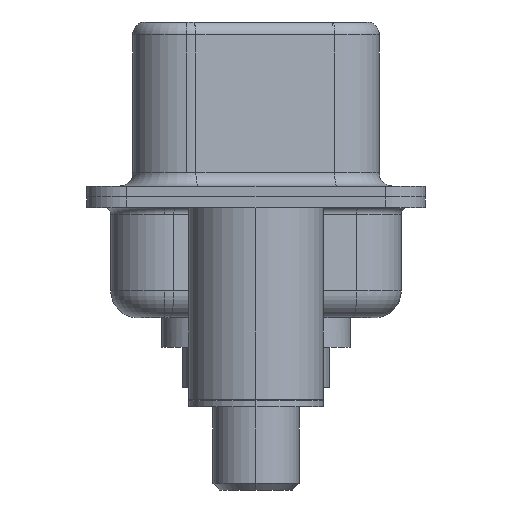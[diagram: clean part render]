
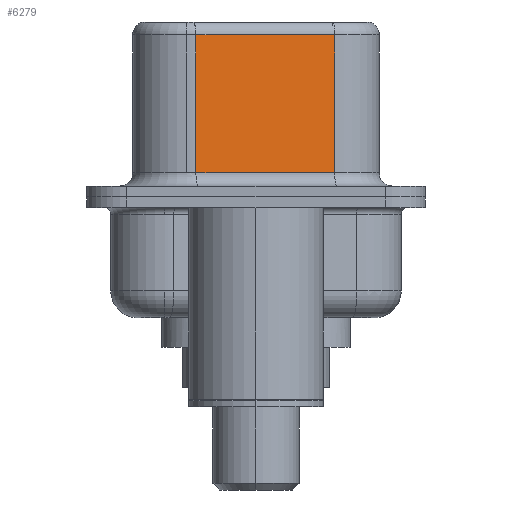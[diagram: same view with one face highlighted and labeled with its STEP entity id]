
A CAD part, left-side view. The second image highlights one B-rep face of the part: STEP entity #6279.
In plain terms, the highlighted planar face has unit normal (-0.985, -0.174, 0).
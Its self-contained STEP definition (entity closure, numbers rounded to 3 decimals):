
#723 = ORIENTED_EDGE ( 'NONE', *, *, #12810, .T. ) ;
#976 = AXIS2_PLACEMENT_3D ( 'NONE', #3949, #3891, #9021 ) ;
#1210 = CARTESIAN_POINT ( 'NONE',  ( 3.67, 2.233, 6.52 ) ) ;
#2506 = EDGE_LOOP ( 'NONE', ( #10487, #8328, #10010, #723 ) ) ;
#3475 = VECTOR ( 'NONE', #10980, 1000. ) ;
#3891 = DIRECTION ( 'NONE',  ( 0.985, 0.174, 0. ) ) ;
#3949 = CARTESIAN_POINT ( 'NONE',  ( 4.58, -2.927, 6.52 ) ) ;
#4405 = DIRECTION ( 'NONE',  ( 0., 0., -1. ) ) ;
#4827 = LINE ( 'NONE', #1210, #15262 ) ;
#5001 = DIRECTION ( 'NONE',  ( 0., 0., -1. ) ) ;
#5284 = VERTEX_POINT ( 'NONE', #11114 ) ;
#5422 = VERTEX_POINT ( 'NONE', #15187 ) ;
#6279 = ADVANCED_FACE ( 'NONE', ( #13656 ), #7757, .F. ) ;
#6617 = VECTOR ( 'NONE', #4405, 1000. ) ;
#6735 = CARTESIAN_POINT ( 'NONE',  ( 4.58, -2.927, 0.9 ) ) ;
#7038 = LINE ( 'NONE', #6735, #13051 ) ;
#7645 = EDGE_CURVE ( 'NONE', #5284, #5422, #10039, .T. ) ;
#7757 = PLANE ( 'NONE',  #976 ) ;
#8038 = CARTESIAN_POINT ( 'NONE',  ( 4.58, -2.927, 6.52 ) ) ;
#8328 = ORIENTED_EDGE ( 'NONE', *, *, #12113, .T. ) ;
#9021 = DIRECTION ( 'NONE',  ( -0.174, 0.985, 0. ) ) ;
#10010 = ORIENTED_EDGE ( 'NONE', *, *, #13079, .T. ) ;
#10039 = LINE ( 'NONE', #8038, #6617 ) ;
#10487 = ORIENTED_EDGE ( 'NONE', *, *, #7645, .F. ) ;
#10980 = DIRECTION ( 'NONE',  ( -0.174, 0.985, 0. ) ) ;
#11114 = CARTESIAN_POINT ( 'NONE',  ( 4.58, -2.927, 6.02 ) ) ;
#11416 = CARTESIAN_POINT ( 'NONE',  ( 3.67, 2.233, 6.02 ) ) ;
#11634 = VERTEX_POINT ( 'NONE', #11416 ) ;
#12113 = EDGE_CURVE ( 'NONE', #5284, #11634, #16291, .T. ) ;
#12155 = CARTESIAN_POINT ( 'NONE',  ( 4.58, -2.927, 6.02 ) ) ;
#12810 = EDGE_CURVE ( 'NONE', #12925, #5422, #7038, .T. ) ;
#12925 = VERTEX_POINT ( 'NONE', #15822 ) ;
#13026 = DIRECTION ( 'NONE',  ( 0.174, -0.985, 0. ) ) ;
#13051 = VECTOR ( 'NONE', #13026, 1000. ) ;
#13079 = EDGE_CURVE ( 'NONE', #11634, #12925, #4827, .T. ) ;
#13656 = FACE_OUTER_BOUND ( 'NONE', #2506, .T. ) ;
#15187 = CARTESIAN_POINT ( 'NONE',  ( 4.58, -2.927, 0.9 ) ) ;
#15262 = VECTOR ( 'NONE', #5001, 1000. ) ;
#15822 = CARTESIAN_POINT ( 'NONE',  ( 3.67, 2.233, 0.9 ) ) ;
#16291 = LINE ( 'NONE', #12155, #3475 ) ;
